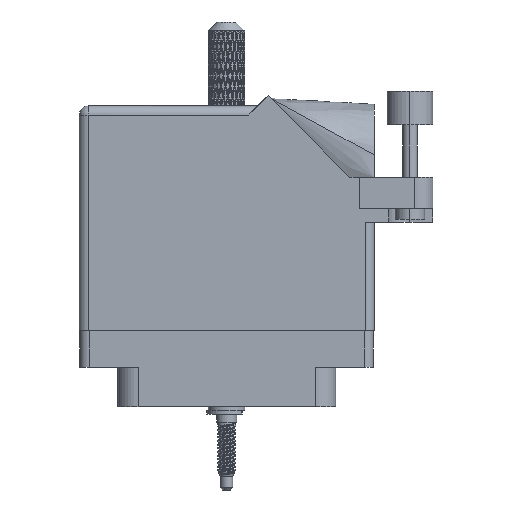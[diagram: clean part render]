
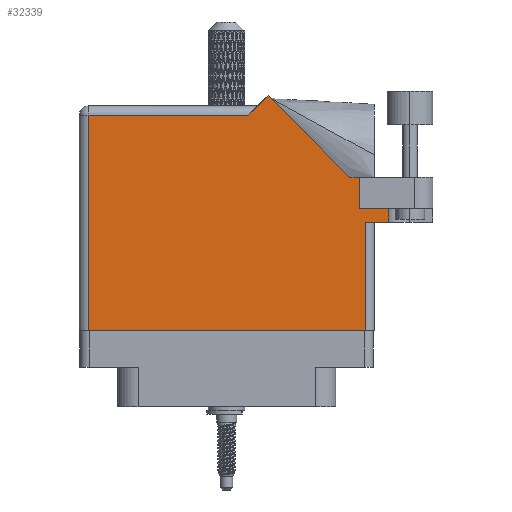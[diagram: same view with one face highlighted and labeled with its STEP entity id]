
A CAD part, front view. The second image highlights one B-rep face of the part: STEP entity #32339.
In plain terms, the highlighted face is planar.
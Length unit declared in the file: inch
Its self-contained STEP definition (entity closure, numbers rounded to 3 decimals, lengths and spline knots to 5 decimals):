
#1087 = ORIENTED_EDGE ( 'NONE', *, *, #80355, .T. ) ;
#3357 = CARTESIAN_POINT ( 'NONE',  ( 0.905, 0.731, 0.455 ) ) ;
#4209 = LINE ( 'NONE', #95882, #54217 ) ;
#4435 = CARTESIAN_POINT ( 'NONE',  ( 0.905, 0.731, 0.455 ) ) ;
#4729 = EDGE_LOOP ( 'NONE', ( #1087, #97229, #53450, #94191, #44136, #43878, #63817, #47486, #85705, #40338, #25421 ) ) ;
#8583 = EDGE_CURVE ( 'NONE', #95283, #43844, #55893, .T. ) ;
#8724 = CARTESIAN_POINT ( 'NONE',  ( 0.943, -0.1, 0.455 ) ) ;
#9656 = CARTESIAN_POINT ( 'NONE',  ( 1.1065, 1.06177, 0.455 ) ) ;
#10595 = LINE ( 'NONE', #84235, #18279 ) ;
#11330 = LINE ( 'NONE', #60404, #94737 ) ;
#11404 = DIRECTION ( 'NONE',  ( -1., 0., 0. ) ) ;
#11543 = DIRECTION ( 'NONE',  ( 1., 0., 0. ) ) ;
#11673 = DIRECTION ( 'NONE',  ( 0., 1., 0. ) ) ;
#14084 = EDGE_CURVE ( 'NONE', #87490, #65885, #20303, .T. ) ;
#17406 = VECTOR ( 'NONE', #11543, 39.37008 ) ;
#18170 = CARTESIAN_POINT ( 'NONE',  ( 0.943, 0.637, 0.455 ) ) ;
#18180 = VECTOR ( 'NONE', #27109, 39.37008 ) ;
#18279 = VECTOR ( 'NONE', #92473, 39.37008 ) ;
#19302 = VECTOR ( 'NONE', #100632, 39.37008 ) ;
#20303 = LINE ( 'NONE', #93413, #69039 ) ;
#22832 = LINE ( 'NONE', #3357, #72856 ) ;
#25421 = ORIENTED_EDGE ( 'NONE', *, *, #31415, .T. ) ;
#26474 = AXIS2_PLACEMENT_3D ( 'NONE', #74605, #99281, #76017 ) ;
#26512 = EDGE_CURVE ( 'NONE', #34349, #31961, #90772, .T. ) ;
#26978 = CARTESIAN_POINT ( 'NONE',  ( -0.943, 1.368, 0.455 ) ) ;
#27109 = DIRECTION ( 'NONE',  ( 0., 1., 0. ) ) ;
#31415 = EDGE_CURVE ( 'NONE', #31961, #89109, #104243, .T. ) ;
#31961 = VERTEX_POINT ( 'NONE', #26978 ) ;
#32269 = DIRECTION ( 'NONE',  ( 0., -1., 0. ) ) ;
#32339 = ADVANCED_FACE ( 'NONE', ( #100247 ), #90689, .F. ) ;
#34349 = VERTEX_POINT ( 'NONE', #62278 ) ;
#38074 = VERTEX_POINT ( 'NONE', #57459 ) ;
#40338 = ORIENTED_EDGE ( 'NONE', *, *, #26512, .T. ) ;
#41922 = EDGE_CURVE ( 'NONE', #38074, #51225, #4209, .T. ) ;
#43844 = VERTEX_POINT ( 'NONE', #101468 ) ;
#43878 = ORIENTED_EDGE ( 'NONE', *, *, #14084, .T. ) ;
#44136 = ORIENTED_EDGE ( 'NONE', *, *, #78672, .F. ) ;
#44153 = CARTESIAN_POINT ( 'NONE',  ( 1.005, 0.637, 0.455 ) ) ;
#44593 = VECTOR ( 'NONE', #11404, 39.37008 ) ;
#45310 = DIRECTION ( 'NONE',  ( 1., 0., 0. ) ) ;
#46151 = EDGE_CURVE ( 'NONE', #51225, #34349, #11330, .T. ) ;
#47486 = ORIENTED_EDGE ( 'NONE', *, *, #41922, .T. ) ;
#48440 = CARTESIAN_POINT ( 'NONE',  ( -0.943, -0.1, 0.455 ) ) ;
#51225 = VERTEX_POINT ( 'NONE', #59887 ) ;
#52788 = CARTESIAN_POINT ( 'NONE',  ( 0.943, 0.637, 0.455 ) ) ;
#53349 = CARTESIAN_POINT ( 'NONE',  ( -1.005, 1.368, 0.455 ) ) ;
#53450 = ORIENTED_EDGE ( 'NONE', *, *, #8583, .T. ) ;
#54217 = VECTOR ( 'NONE', #104054, 39.37008 ) ;
#55893 = LINE ( 'NONE', #44153, #17406 ) ;
#56782 = CARTESIAN_POINT ( 'NONE',  ( 1.1065, 0.731, 0.455 ) ) ;
#57459 = CARTESIAN_POINT ( 'NONE',  ( 0.83942, 0.944, 0.455 ) ) ;
#59232 = LINE ( 'NONE', #18170, #18180 ) ;
#59887 = CARTESIAN_POINT ( 'NONE',  ( 0.28271, 1.50071, 0.455 ) ) ;
#60404 = CARTESIAN_POINT ( 'NONE',  ( 0.212, 1.43, 0.455 ) ) ;
#60508 = CARTESIAN_POINT ( 'NONE',  ( -0.943, -0.1, 0.455 ) ) ;
#60748 = EDGE_CURVE ( 'NONE', #65885, #38074, #10595, .T. ) ;
#61191 = EDGE_CURVE ( 'NONE', #81067, #95283, #59232, .T. ) ;
#62278 = CARTESIAN_POINT ( 'NONE',  ( 0.15, 1.368, 0.455 ) ) ;
#63817 = ORIENTED_EDGE ( 'NONE', *, *, #60748, .T. ) ;
#65885 = VERTEX_POINT ( 'NONE', #78758 ) ;
#69039 = VECTOR ( 'NONE', #11673, 39.37008 ) ;
#72856 = VECTOR ( 'NONE', #45310, 39.37008 ) ;
#74605 = CARTESIAN_POINT ( 'NONE',  ( -1.005, 1.43, 0.455 ) ) ;
#74956 = EDGE_CURVE ( 'NONE', #93534, #43844, #83503, .T. ) ;
#76017 = DIRECTION ( 'NONE',  ( -1., 0., 0. ) ) ;
#78672 = EDGE_CURVE ( 'NONE', #87490, #93534, #22832, .T. ) ;
#78758 = CARTESIAN_POINT ( 'NONE',  ( 0.905, 0.944, 0.455 ) ) ;
#80355 = EDGE_CURVE ( 'NONE', #89109, #81067, #86717, .T. ) ;
#81067 = VERTEX_POINT ( 'NONE', #8724 ) ;
#81334 = CARTESIAN_POINT ( 'NONE',  ( -1.005, -0.1, 0.455 ) ) ;
#83503 = LINE ( 'NONE', #9656, #19302 ) ;
#84235 = CARTESIAN_POINT ( 'NONE',  ( 1.405, 0.944, 0.455 ) ) ;
#85705 = ORIENTED_EDGE ( 'NONE', *, *, #46151, .T. ) ;
#86717 = LINE ( 'NONE', #81334, #97031 ) ;
#87490 = VERTEX_POINT ( 'NONE', #4435 ) ;
#87626 = VECTOR ( 'NONE', #32269, 39.37008 ) ;
#89109 = VERTEX_POINT ( 'NONE', #60508 ) ;
#90689 = PLANE ( 'NONE',  #26474 ) ;
#90772 = LINE ( 'NONE', #53349, #44593 ) ;
#92473 = DIRECTION ( 'NONE',  ( -1., 0., 0. ) ) ;
#93413 = CARTESIAN_POINT ( 'NONE',  ( 0.905, 0.731, 0.455 ) ) ;
#93534 = VERTEX_POINT ( 'NONE', #56782 ) ;
#94191 = ORIENTED_EDGE ( 'NONE', *, *, #74956, .F. ) ;
#94737 = VECTOR ( 'NONE', #100892, 39.37008 ) ;
#95283 = VERTEX_POINT ( 'NONE', #52788 ) ;
#95882 = CARTESIAN_POINT ( 'NONE',  ( 0.83942, 0.944, 0.455 ) ) ;
#97031 = VECTOR ( 'NONE', #105657, 39.37008 ) ;
#97229 = ORIENTED_EDGE ( 'NONE', *, *, #61191, .T. ) ;
#99281 = DIRECTION ( 'NONE',  ( 0., 0., -1. ) ) ;
#100247 = FACE_OUTER_BOUND ( 'NONE', #4729, .T. ) ;
#100632 = DIRECTION ( 'NONE',  ( 0., -1., 0. ) ) ;
#100892 = DIRECTION ( 'NONE',  ( -0.707, -0.707, 0. ) ) ;
#101468 = CARTESIAN_POINT ( 'NONE',  ( 1.1065, 0.637, 0.455 ) ) ;
#104054 = DIRECTION ( 'NONE',  ( -0.707, 0.707, 0. ) ) ;
#104243 = LINE ( 'NONE', #48440, #87626 ) ;
#105657 = DIRECTION ( 'NONE',  ( 1., 0., 0. ) ) ;
